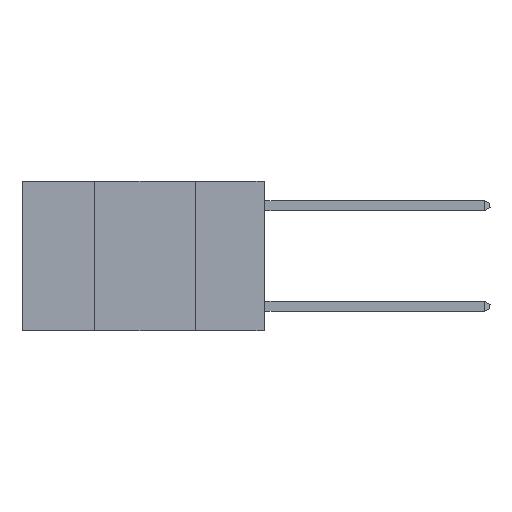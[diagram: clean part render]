
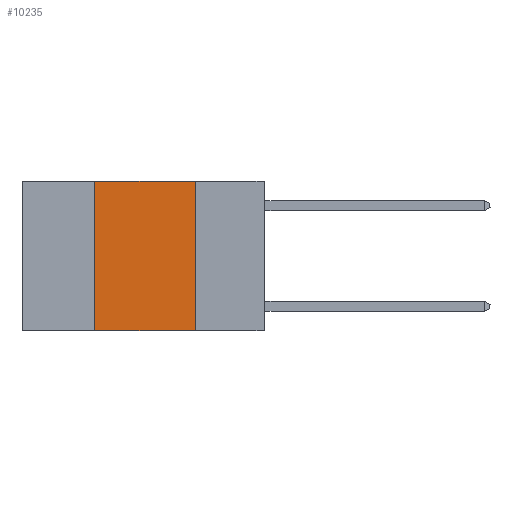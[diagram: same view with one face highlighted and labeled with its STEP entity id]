
A CAD part, left-side view. The second image highlights one B-rep face of the part: STEP entity #10235.
In plain terms, the highlighted planar face has unit normal (-1, 0, 0).
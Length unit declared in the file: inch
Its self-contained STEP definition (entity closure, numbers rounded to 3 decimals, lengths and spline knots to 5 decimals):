
#109 = CARTESIAN_POINT ( 'NONE',  ( 0., 0.6, 0. ) ) ;
#135 = AXIS2_PLACEMENT_3D ( 'NONE', #5842, #5664, #9464 ) ;
#263 = CARTESIAN_POINT ( 'NONE',  ( 0., 0.42, 0. ) ) ;
#462 = CARTESIAN_POINT ( 'NONE',  ( 0., 0.42, -0.37 ) ) ;
#1299 = VECTOR ( 'NONE', #8717, 39.37008 ) ;
#2076 = VECTOR ( 'NONE', #11391, 39.37008 ) ;
#2127 = DIRECTION ( 'NONE',  ( 0., 0., -1. ) ) ;
#2368 = LINE ( 'NONE', #8581, #2470 ) ;
#2470 = VECTOR ( 'NONE', #2127, 39.37008 ) ;
#2823 = EDGE_CURVE ( 'NONE', #7484, #7994, #9326, .T. ) ;
#2942 = CARTESIAN_POINT ( 'NONE',  ( 0., 0.6, -0.37 ) ) ;
#2992 = ORIENTED_EDGE ( 'NONE', *, *, #7626, .F. ) ;
#3857 = ORIENTED_EDGE ( 'NONE', *, *, #7932, .F. ) ;
#3883 = EDGE_CURVE ( 'NONE', #7484, #6696, #10374, .T. ) ;
#4081 = EDGE_LOOP ( 'NONE', ( #3857, #2992, #9717, #6074 ) ) ;
#4794 = VERTEX_POINT ( 'NONE', #9245 ) ;
#5664 = DIRECTION ( 'NONE',  ( 1., 0., 0. ) ) ;
#5842 = CARTESIAN_POINT ( 'NONE',  ( 0., 0.6, 0. ) ) ;
#6074 = ORIENTED_EDGE ( 'NONE', *, *, #3883, .T. ) ;
#6121 = VECTOR ( 'NONE', #10308, 39.37008 ) ;
#6696 = VERTEX_POINT ( 'NONE', #9113 ) ;
#7453 = PLANE ( 'NONE',  #135 ) ;
#7484 = VERTEX_POINT ( 'NONE', #462 ) ;
#7626 = EDGE_CURVE ( 'NONE', #7994, #4794, #8348, .T. ) ;
#7932 = EDGE_CURVE ( 'NONE', #4794, #6696, #2368, .T. ) ;
#7994 = VERTEX_POINT ( 'NONE', #11565 ) ;
#8348 = LINE ( 'NONE', #109, #1299 ) ;
#8581 = CARTESIAN_POINT ( 'NONE',  ( 0., 0.17, 0. ) ) ;
#8717 = DIRECTION ( 'NONE',  ( 0., -1., 0. ) ) ;
#9113 = CARTESIAN_POINT ( 'NONE',  ( 0., 0.17, -0.37 ) ) ;
#9245 = CARTESIAN_POINT ( 'NONE',  ( 0., 0.17, 0. ) ) ;
#9287 = FACE_OUTER_BOUND ( 'NONE', #4081, .T. ) ;
#9326 = LINE ( 'NONE', #263, #2076 ) ;
#9464 = DIRECTION ( 'NONE',  ( 0., 0., -1. ) ) ;
#9717 = ORIENTED_EDGE ( 'NONE', *, *, #2823, .F. ) ;
#10235 = ADVANCED_FACE ( 'NONE', ( #9287 ), #7453, .F. ) ;
#10308 = DIRECTION ( 'NONE',  ( 0., -1., 0. ) ) ;
#10374 = LINE ( 'NONE', #2942, #6121 ) ;
#11391 = DIRECTION ( 'NONE',  ( 0., 0., 1. ) ) ;
#11565 = CARTESIAN_POINT ( 'NONE',  ( 0., 0.42, 0. ) ) ;
